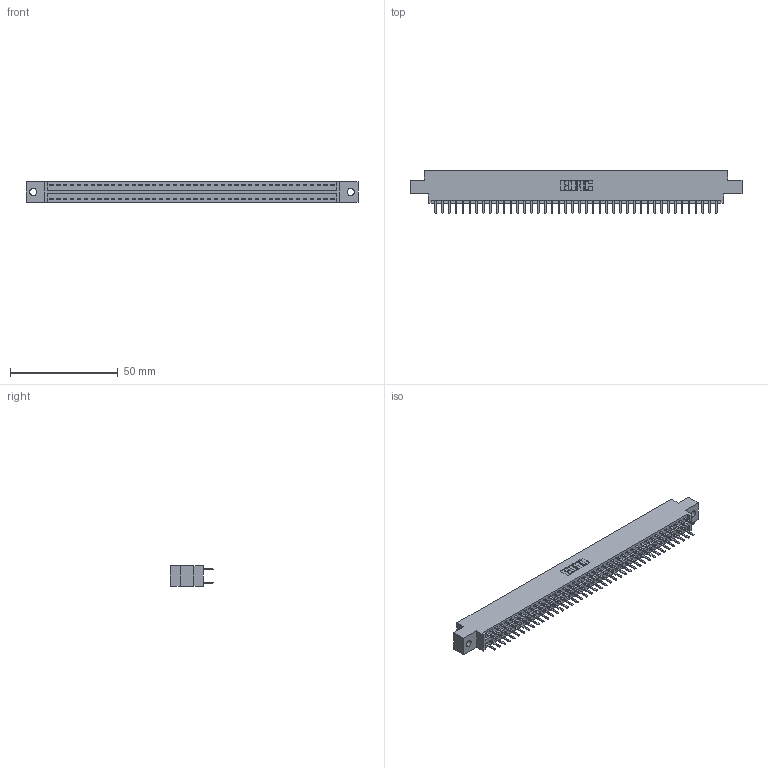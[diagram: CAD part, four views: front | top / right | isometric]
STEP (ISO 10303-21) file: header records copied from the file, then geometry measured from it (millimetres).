
FILE_DESCRIPTION (( 'STEP AP203' ), '1' );
FILE_NAME ('346-084-520-802.STEP', '2018-08-29T10:49:37', ( '' ), ( '' ), 'SwSTEP 2.0', 'SolidWorks 2016', '' );
FILE_SCHEMA (( 'CONFIG_CONTROL_DESIGN' ));
Length unit declared in the file: inch
Products named in the file (3): 346 Part_0.170 Offset - 0.128 Dia; 345-292-001_345-293-120; 346-084-520-802
Assembly tree (85 placements, depth 2):
  346-084-520-802
    346 Part_0.170 Offset - 0.128 Dia
    345-292-001_345-293-120  x84
Bounding box: 153.92 x 20.02 x 9.4 mm (x, y, z)
Volume: 14781.3 mm3; surface area: 20141.7 mm2
Topology: 85 solids, 85 shells, 4830 faces, 14033 edges, 9130 vertices
Faces by surface type: plane 3188, cylinder 1642
Entity records: 27659 total; most frequent: CARTESIAN_POINT 4572, ORIENTED_EDGE 4494, DIRECTION 4067, EDGE_CURVE 2247, LINE 1943, VECTOR 1943, VERTEX_POINT 1494, AXIS2_PLACEMENT_3D 1062
